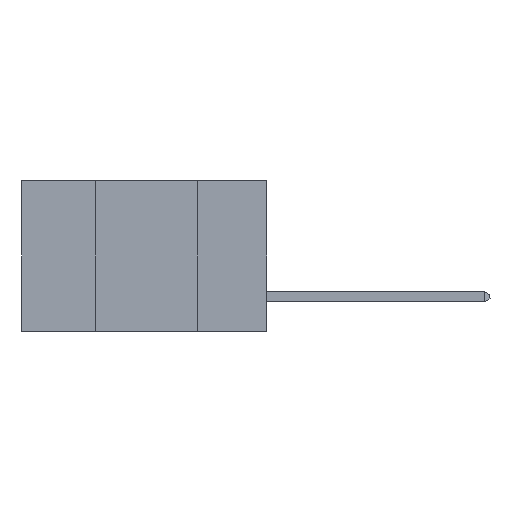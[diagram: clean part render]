
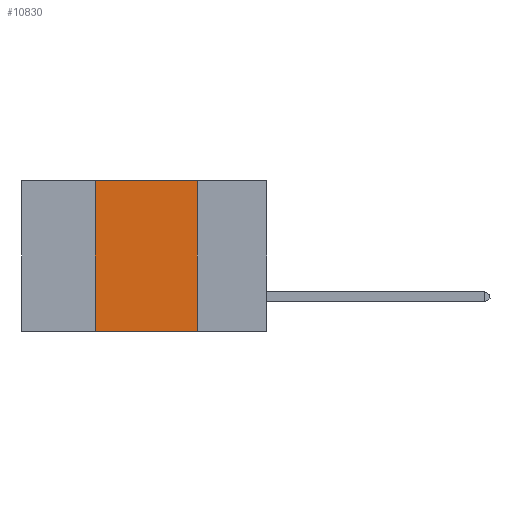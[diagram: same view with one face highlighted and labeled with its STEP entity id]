
A CAD part, left-side view. The second image highlights one B-rep face of the part: STEP entity #10830.
In plain terms, the highlighted planar face has unit normal (-1, 0, 0).
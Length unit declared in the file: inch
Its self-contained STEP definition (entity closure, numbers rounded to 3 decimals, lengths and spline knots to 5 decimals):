
#1076 = VECTOR ( 'NONE', #7531, 39.37008 ) ;
#2011 = CARTESIAN_POINT ( 'NONE',  ( 0., 0.6, -0.37 ) ) ;
#2766 = CARTESIAN_POINT ( 'NONE',  ( 0., 0.42, 0. ) ) ;
#3532 = CARTESIAN_POINT ( 'NONE',  ( 0., 0.17, 0. ) ) ;
#3768 = AXIS2_PLACEMENT_3D ( 'NONE', #18589, #9415, #22193 ) ;
#4196 = VECTOR ( 'NONE', #4590, 39.37008 ) ;
#4590 = DIRECTION ( 'NONE',  ( 0., 0., 1. ) ) ;
#4931 = LINE ( 'NONE', #3532, #14198 ) ;
#6495 = LINE ( 'NONE', #17823, #10305 ) ;
#6734 = DIRECTION ( 'NONE',  ( 0., -1., 0. ) ) ;
#7298 = CARTESIAN_POINT ( 'NONE',  ( 0., 0.17, -0.37 ) ) ;
#7348 = ORIENTED_EDGE ( 'NONE', *, *, #22074, .F. ) ;
#7507 = PLANE ( 'NONE',  #3768 ) ;
#7531 = DIRECTION ( 'NONE',  ( 0., -1., 0. ) ) ;
#8393 = VERTEX_POINT ( 'NONE', #15179 ) ;
#8551 = EDGE_CURVE ( 'NONE', #19660, #12644, #14577, .T. ) ;
#8592 = FACE_OUTER_BOUND ( 'NONE', #12870, .T. ) ;
#9080 = DIRECTION ( 'NONE',  ( 0., 0., -1. ) ) ;
#9415 = DIRECTION ( 'NONE',  ( 1., 0., 0. ) ) ;
#10123 = VERTEX_POINT ( 'NONE', #7298 ) ;
#10305 = VECTOR ( 'NONE', #6734, 39.37008 ) ;
#10830 = ADVANCED_FACE ( 'NONE', ( #8592 ), #7507, .F. ) ;
#11175 = EDGE_CURVE ( 'NONE', #19660, #10123, #15836, .T. ) ;
#11179 = ORIENTED_EDGE ( 'NONE', *, *, #18272, .F. ) ;
#12644 = VERTEX_POINT ( 'NONE', #15863 ) ;
#12870 = EDGE_LOOP ( 'NONE', ( #11179, #7348, #12892, #23651 ) ) ;
#12892 = ORIENTED_EDGE ( 'NONE', *, *, #8551, .F. ) ;
#14198 = VECTOR ( 'NONE', #9080, 39.37008 ) ;
#14577 = LINE ( 'NONE', #2766, #4196 ) ;
#15179 = CARTESIAN_POINT ( 'NONE',  ( 0., 0.17, 0. ) ) ;
#15836 = LINE ( 'NONE', #2011, #1076 ) ;
#15863 = CARTESIAN_POINT ( 'NONE',  ( 0., 0.42, 0. ) ) ;
#16852 = CARTESIAN_POINT ( 'NONE',  ( 0., 0.42, -0.37 ) ) ;
#17823 = CARTESIAN_POINT ( 'NONE',  ( 0., 0.6, 0. ) ) ;
#18272 = EDGE_CURVE ( 'NONE', #8393, #10123, #4931, .T. ) ;
#18589 = CARTESIAN_POINT ( 'NONE',  ( 0., 0.6, 0. ) ) ;
#19660 = VERTEX_POINT ( 'NONE', #16852 ) ;
#22074 = EDGE_CURVE ( 'NONE', #12644, #8393, #6495, .T. ) ;
#22193 = DIRECTION ( 'NONE',  ( 0., 0., -1. ) ) ;
#23651 = ORIENTED_EDGE ( 'NONE', *, *, #11175, .T. ) ;
